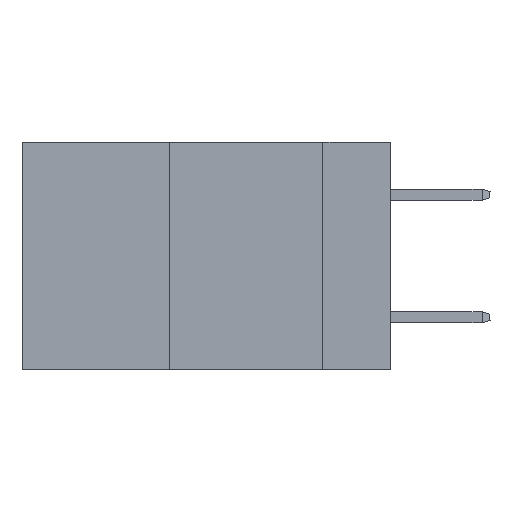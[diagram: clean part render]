
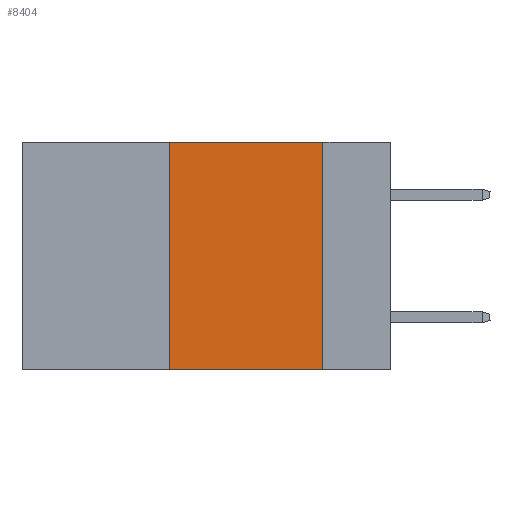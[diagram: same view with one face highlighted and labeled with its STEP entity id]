
A CAD part, left-side view. The second image highlights one B-rep face of the part: STEP entity #8404.
In plain terms, the highlighted planar face has unit normal (-1, 0, 0).
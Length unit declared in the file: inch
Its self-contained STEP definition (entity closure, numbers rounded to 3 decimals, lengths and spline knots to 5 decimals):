
#71 = VERTEX_POINT ( 'NONE', #7191 ) ;
#728 = DIRECTION ( 'NONE',  ( 1., 0., 0. ) ) ;
#1472 = CARTESIAN_POINT ( 'NONE',  ( 0., 0.11, -0.37 ) ) ;
#1476 = VERTEX_POINT ( 'NONE', #1472 ) ;
#4074 = VECTOR ( 'NONE', #5984, 39.37008 ) ;
#5320 = LINE ( 'NONE', #6295, #17700 ) ;
#5959 = ORIENTED_EDGE ( 'NONE', *, *, #14803, .F. ) ;
#5984 = DIRECTION ( 'NONE',  ( 0., -1., 0. ) ) ;
#6239 = CARTESIAN_POINT ( 'NONE',  ( 0., 0.6, 0. ) ) ;
#6295 = CARTESIAN_POINT ( 'NONE',  ( 0., 0.11, 0. ) ) ;
#7030 = CARTESIAN_POINT ( 'NONE',  ( 0., 0.36, 0. ) ) ;
#7191 = CARTESIAN_POINT ( 'NONE',  ( 0., 0.36, 0. ) ) ;
#8404 = ADVANCED_FACE ( 'NONE', ( #16958 ), #27710, .F. ) ;
#9386 = AXIS2_PLACEMENT_3D ( 'NONE', #30118, #728, #18101 ) ;
#10218 = EDGE_CURVE ( 'NONE', #23731, #1476, #22961, .T. ) ;
#11042 = LINE ( 'NONE', #7030, #17555 ) ;
#11171 = CARTESIAN_POINT ( 'NONE',  ( 0., 0.11, 0. ) ) ;
#11234 = DIRECTION ( 'NONE',  ( 0., -1., 0. ) ) ;
#11280 = DIRECTION ( 'NONE',  ( 0., 0., -1. ) ) ;
#11626 = VECTOR ( 'NONE', #11234, 39.37008 ) ;
#14803 = EDGE_CURVE ( 'NONE', #71, #24012, #30961, .T. ) ;
#16958 = FACE_OUTER_BOUND ( 'NONE', #23810, .T. ) ;
#17555 = VECTOR ( 'NONE', #24166, 39.37008 ) ;
#17657 = EDGE_CURVE ( 'NONE', #23731, #71, #11042, .T. ) ;
#17700 = VECTOR ( 'NONE', #11280, 39.37008 ) ;
#18101 = DIRECTION ( 'NONE',  ( 0., 0., -1. ) ) ;
#19424 = ORIENTED_EDGE ( 'NONE', *, *, #27374, .F. ) ;
#21688 = ORIENTED_EDGE ( 'NONE', *, *, #10218, .T. ) ;
#22961 = LINE ( 'NONE', #27875, #4074 ) ;
#23731 = VERTEX_POINT ( 'NONE', #29524 ) ;
#23810 = EDGE_LOOP ( 'NONE', ( #19424, #5959, #29193, #21688 ) ) ;
#24012 = VERTEX_POINT ( 'NONE', #11171 ) ;
#24166 = DIRECTION ( 'NONE',  ( 0., 0., 1. ) ) ;
#27374 = EDGE_CURVE ( 'NONE', #24012, #1476, #5320, .T. ) ;
#27710 = PLANE ( 'NONE',  #9386 ) ;
#27875 = CARTESIAN_POINT ( 'NONE',  ( 0., 0.6, -0.37 ) ) ;
#29193 = ORIENTED_EDGE ( 'NONE', *, *, #17657, .F. ) ;
#29524 = CARTESIAN_POINT ( 'NONE',  ( 0., 0.36, -0.37 ) ) ;
#30118 = CARTESIAN_POINT ( 'NONE',  ( 0., 0.6, 0. ) ) ;
#30961 = LINE ( 'NONE', #6239, #11626 ) ;
